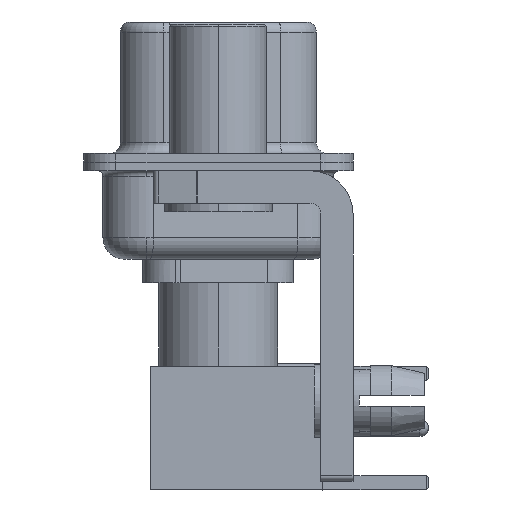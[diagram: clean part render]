
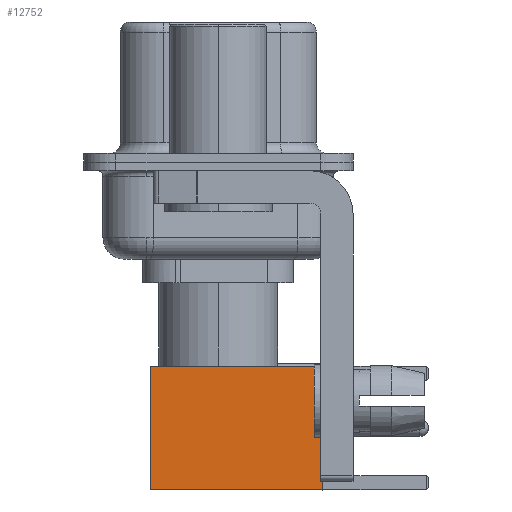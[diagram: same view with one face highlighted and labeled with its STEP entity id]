
A CAD part, left-side view. The second image highlights one B-rep face of the part: STEP entity #12752.
In plain terms, the highlighted face is planar.
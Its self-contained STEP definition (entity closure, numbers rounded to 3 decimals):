
#526 = VECTOR ( 'NONE', #25786, 1000. ) ;
#1046 = VERTEX_POINT ( 'NONE', #13537 ) ;
#1309 = DIRECTION ( 'NONE',  ( 0., 0., 1. ) ) ;
#2813 = VECTOR ( 'NONE', #8458, 1000. ) ;
#2962 = DIRECTION ( 'NONE',  ( 0., 0., -1. ) ) ;
#3138 = LINE ( 'NONE', #20940, #31879 ) ;
#3277 = CARTESIAN_POINT ( 'NONE',  ( -2.875, 2.875, 0. ) ) ;
#6146 = CARTESIAN_POINT ( 'NONE',  ( -2.875, 2.875, 8. ) ) ;
#6819 = CARTESIAN_POINT ( 'NONE',  ( 2.875, 2.875, 0. ) ) ;
#8458 = DIRECTION ( 'NONE',  ( 0., 0., -1. ) ) ;
#12752 = ADVANCED_FACE ( 'NONE', ( #25318 ), #14093, .T. ) ;
#12819 = LINE ( 'NONE', #23364, #526 ) ;
#13537 = CARTESIAN_POINT ( 'NONE',  ( 2.875, 2.875, 0. ) ) ;
#13815 = EDGE_CURVE ( 'NONE', #29112, #1046, #3138, .T. ) ;
#14093 = PLANE ( 'NONE',  #25562 ) ;
#14320 = EDGE_LOOP ( 'NONE', ( #31108, #18523, #30273, #25250 ) ) ;
#14521 = VECTOR ( 'NONE', #22183, 1000. ) ;
#17288 = EDGE_CURVE ( 'NONE', #29112, #33049, #12819, .T. ) ;
#18523 = ORIENTED_EDGE ( 'NONE', *, *, #33596, .T. ) ;
#20940 = CARTESIAN_POINT ( 'NONE',  ( 2.875, 2.875, 0. ) ) ;
#21763 = LINE ( 'NONE', #3277, #2813 ) ;
#22183 = DIRECTION ( 'NONE',  ( -1., 0., 0. ) ) ;
#22189 = VERTEX_POINT ( 'NONE', #25139 ) ;
#23364 = CARTESIAN_POINT ( 'NONE',  ( 0., 2.875, 8. ) ) ;
#24774 = LINE ( 'NONE', #30130, #14521 ) ;
#24813 = DIRECTION ( 'NONE',  ( 0., 1., 0. ) ) ;
#25139 = CARTESIAN_POINT ( 'NONE',  ( -2.875, 2.875, 0. ) ) ;
#25250 = ORIENTED_EDGE ( 'NONE', *, *, #17288, .F. ) ;
#25318 = FACE_OUTER_BOUND ( 'NONE', #14320, .T. ) ;
#25562 = AXIS2_PLACEMENT_3D ( 'NONE', #6819, #24813, #1309 ) ;
#25786 = DIRECTION ( 'NONE',  ( -1., 0., 0. ) ) ;
#28670 = CARTESIAN_POINT ( 'NONE',  ( 2.875, 2.875, 8. ) ) ;
#29112 = VERTEX_POINT ( 'NONE', #28670 ) ;
#30130 = CARTESIAN_POINT ( 'NONE',  ( 0., 2.875, 0. ) ) ;
#30273 = ORIENTED_EDGE ( 'NONE', *, *, #31206, .F. ) ;
#31108 = ORIENTED_EDGE ( 'NONE', *, *, #13815, .T. ) ;
#31206 = EDGE_CURVE ( 'NONE', #33049, #22189, #21763, .T. ) ;
#31879 = VECTOR ( 'NONE', #2962, 1000. ) ;
#33049 = VERTEX_POINT ( 'NONE', #6146 ) ;
#33596 = EDGE_CURVE ( 'NONE', #1046, #22189, #24774, .T. ) ;
